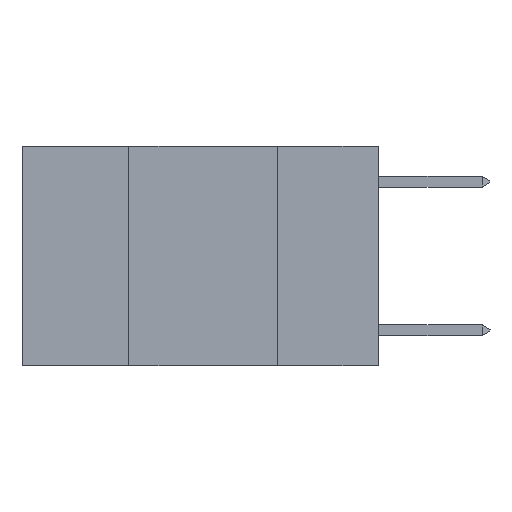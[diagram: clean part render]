
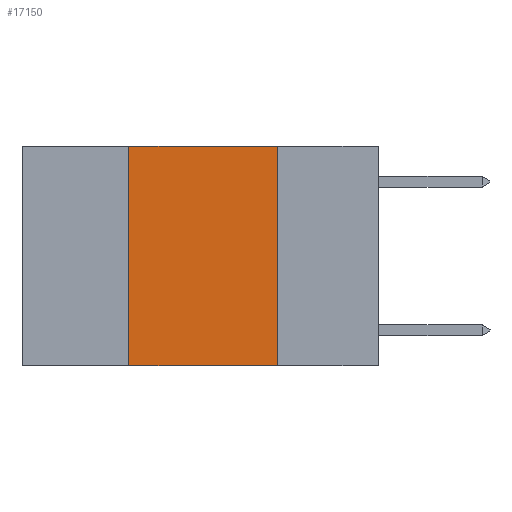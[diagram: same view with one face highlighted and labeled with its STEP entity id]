
A CAD part, left-side view. The second image highlights one B-rep face of the part: STEP entity #17150.
In plain terms, the highlighted planar face has unit normal (-1, 0, 0).
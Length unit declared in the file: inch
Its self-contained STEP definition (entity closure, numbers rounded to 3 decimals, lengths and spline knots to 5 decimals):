
#326 = VERTEX_POINT ( 'NONE', #13275 ) ;
#357 = DIRECTION ( 'NONE',  ( 0., 0., -1. ) ) ;
#580 = CARTESIAN_POINT ( 'NONE',  ( 0., 0.42, 0. ) ) ;
#1400 = CARTESIAN_POINT ( 'NONE',  ( 0., 0.17, -0.37 ) ) ;
#2874 = VECTOR ( 'NONE', #18699, 39.37008 ) ;
#3021 = LINE ( 'NONE', #20416, #17284 ) ;
#3615 = CARTESIAN_POINT ( 'NONE',  ( 0., 0.42, -0.37 ) ) ;
#3832 = CARTESIAN_POINT ( 'NONE',  ( 0., 0.6, 0. ) ) ;
#4216 = DIRECTION ( 'NONE',  ( 0., 0., 1. ) ) ;
#4370 = LINE ( 'NONE', #20810, #22826 ) ;
#6014 = VECTOR ( 'NONE', #11120, 39.37008 ) ;
#7029 = FACE_OUTER_BOUND ( 'NONE', #13635, .T. ) ;
#7499 = EDGE_CURVE ( 'NONE', #15803, #326, #17737, .T. ) ;
#8154 = AXIS2_PLACEMENT_3D ( 'NONE', #20795, #11683, #357 ) ;
#9183 = ORIENTED_EDGE ( 'NONE', *, *, #23624, .T. ) ;
#9839 = PLANE ( 'NONE',  #8154 ) ;
#10913 = EDGE_CURVE ( 'NONE', #326, #15408, #3021, .T. ) ;
#11120 = DIRECTION ( 'NONE',  ( 0., -1., 0. ) ) ;
#11352 = ORIENTED_EDGE ( 'NONE', *, *, #20822, .F. ) ;
#11683 = DIRECTION ( 'NONE',  ( 1., 0., 0. ) ) ;
#13275 = CARTESIAN_POINT ( 'NONE',  ( 0., 0.17, 0. ) ) ;
#13635 = EDGE_LOOP ( 'NONE', ( #17914, #17826, #11352, #9183 ) ) ;
#15226 = LINE ( 'NONE', #23903, #6014 ) ;
#15408 = VERTEX_POINT ( 'NONE', #1400 ) ;
#15803 = VERTEX_POINT ( 'NONE', #580 ) ;
#17150 = ADVANCED_FACE ( 'NONE', ( #7029 ), #9839, .F. ) ;
#17284 = VECTOR ( 'NONE', #22227, 39.37008 ) ;
#17737 = LINE ( 'NONE', #3832, #2874 ) ;
#17826 = ORIENTED_EDGE ( 'NONE', *, *, #7499, .F. ) ;
#17914 = ORIENTED_EDGE ( 'NONE', *, *, #10913, .F. ) ;
#18699 = DIRECTION ( 'NONE',  ( 0., -1., 0. ) ) ;
#18998 = VERTEX_POINT ( 'NONE', #3615 ) ;
#20416 = CARTESIAN_POINT ( 'NONE',  ( 0., 0.17, 0. ) ) ;
#20795 = CARTESIAN_POINT ( 'NONE',  ( 0., 0.6, 0. ) ) ;
#20810 = CARTESIAN_POINT ( 'NONE',  ( 0., 0.42, 0. ) ) ;
#20822 = EDGE_CURVE ( 'NONE', #18998, #15803, #4370, .T. ) ;
#22227 = DIRECTION ( 'NONE',  ( 0., 0., -1. ) ) ;
#22826 = VECTOR ( 'NONE', #4216, 39.37008 ) ;
#23624 = EDGE_CURVE ( 'NONE', #18998, #15408, #15226, .T. ) ;
#23903 = CARTESIAN_POINT ( 'NONE',  ( 0., 0.6, -0.37 ) ) ;
